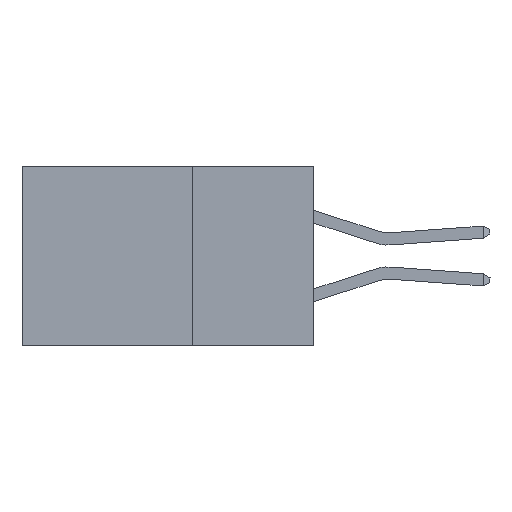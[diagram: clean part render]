
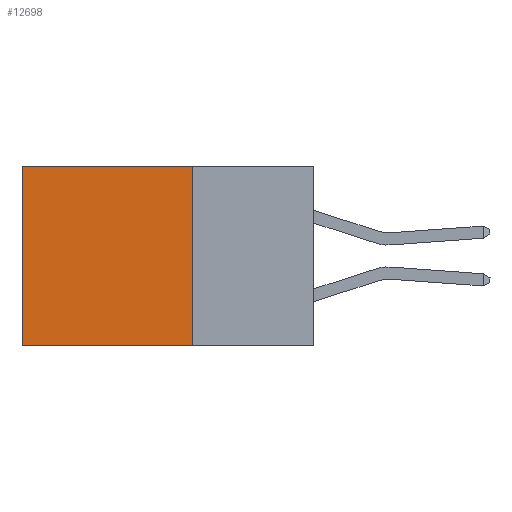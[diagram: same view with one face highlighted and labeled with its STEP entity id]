
A CAD part, left-side view. The second image highlights one B-rep face of the part: STEP entity #12698.
In plain terms, the highlighted planar face has unit normal (-1, 0, 0).
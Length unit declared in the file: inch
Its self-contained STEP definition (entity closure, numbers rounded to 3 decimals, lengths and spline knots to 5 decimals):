
#997 = CARTESIAN_POINT ( 'NONE',  ( 0.2875, 0.6, 0. ) ) ;
#3009 = CARTESIAN_POINT ( 'NONE',  ( 0.2875, 0.25, 0. ) ) ;
#4056 = CARTESIAN_POINT ( 'NONE',  ( 0.2875, 0.25, -0.37 ) ) ;
#4269 = ORIENTED_EDGE ( 'NONE', *, *, #28027, .T. ) ;
#4509 = DIRECTION ( 'NONE',  ( 0., 1., 0. ) ) ;
#4769 = CARTESIAN_POINT ( 'NONE',  ( 0.2875, 0.6, -0.37 ) ) ;
#5054 = EDGE_LOOP ( 'NONE', ( #18117, #29294, #32033, #4269 ) ) ;
#5545 = DIRECTION ( 'NONE',  ( 0., 0., -1. ) ) ;
#5910 = VECTOR ( 'NONE', #4509, 39.37008 ) ;
#7464 = VERTEX_POINT ( 'NONE', #16271 ) ;
#9095 = CARTESIAN_POINT ( 'NONE',  ( 0.2875, 0.25, 0. ) ) ;
#9206 = DIRECTION ( 'NONE',  ( 0., 0., -1. ) ) ;
#10633 = CARTESIAN_POINT ( 'NONE',  ( 0.2875, 0.25, 0. ) ) ;
#12382 = CARTESIAN_POINT ( 'NONE',  ( 0.2875, 0.25, -0.37 ) ) ;
#12698 = ADVANCED_FACE ( 'NONE', ( #28210 ), #23654, .F. ) ;
#13785 = LINE ( 'NONE', #997, #22534 ) ;
#15735 = VERTEX_POINT ( 'NONE', #23887 ) ;
#16271 = CARTESIAN_POINT ( 'NONE',  ( 0.2875, 0.25, 0. ) ) ;
#18117 = ORIENTED_EDGE ( 'NONE', *, *, #24458, .T. ) ;
#18753 = DIRECTION ( 'NONE',  ( 0., 0., -1. ) ) ;
#18924 = LINE ( 'NONE', #9095, #19362 ) ;
#19362 = VECTOR ( 'NONE', #9206, 39.37008 ) ;
#20289 = VECTOR ( 'NONE', #20863, 39.37008 ) ;
#20860 = DIRECTION ( 'NONE',  ( 1., 0., 0. ) ) ;
#20863 = DIRECTION ( 'NONE',  ( 0., 1., 0. ) ) ;
#22534 = VECTOR ( 'NONE', #18753, 39.37008 ) ;
#23043 = LINE ( 'NONE', #3009, #20289 ) ;
#23654 = PLANE ( 'NONE',  #32240 ) ;
#23887 = CARTESIAN_POINT ( 'NONE',  ( 0.2875, 0.6, 0. ) ) ;
#24458 = EDGE_CURVE ( 'NONE', #15735, #28383, #13785, .T. ) ;
#24982 = LINE ( 'NONE', #12382, #5910 ) ;
#28027 = EDGE_CURVE ( 'NONE', #7464, #15735, #23043, .T. ) ;
#28210 = FACE_OUTER_BOUND ( 'NONE', #5054, .T. ) ;
#28383 = VERTEX_POINT ( 'NONE', #4769 ) ;
#28966 = EDGE_CURVE ( 'NONE', #30146, #28383, #24982, .T. ) ;
#29294 = ORIENTED_EDGE ( 'NONE', *, *, #28966, .F. ) ;
#30146 = VERTEX_POINT ( 'NONE', #4056 ) ;
#31212 = EDGE_CURVE ( 'NONE', #7464, #30146, #18924, .T. ) ;
#32033 = ORIENTED_EDGE ( 'NONE', *, *, #31212, .F. ) ;
#32240 = AXIS2_PLACEMENT_3D ( 'NONE', #10633, #20860, #5545 ) ;
